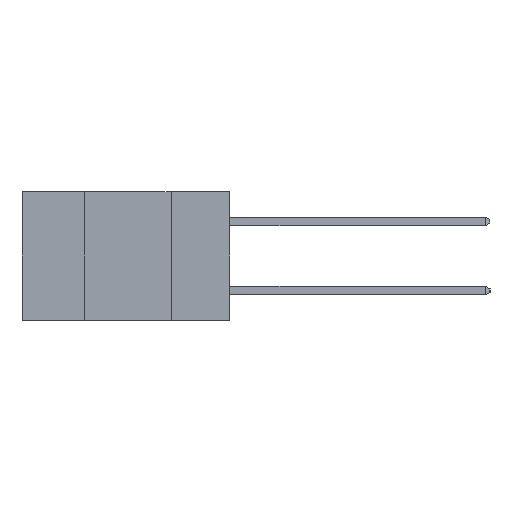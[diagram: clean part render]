
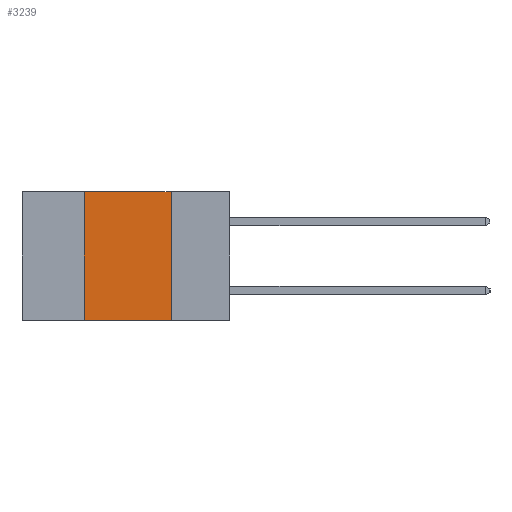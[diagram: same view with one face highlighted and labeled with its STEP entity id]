
A CAD part, left-side view. The second image highlights one B-rep face of the part: STEP entity #3239.
In plain terms, the highlighted planar face has unit normal (-1, 0, 0).
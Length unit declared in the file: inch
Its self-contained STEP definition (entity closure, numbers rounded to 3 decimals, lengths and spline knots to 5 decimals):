
#440 = CARTESIAN_POINT ( 'NONE',  ( 0., 0.42, 0. ) ) ;
#556 = DIRECTION ( 'NONE',  ( 0., 0., 1. ) ) ;
#695 = EDGE_CURVE ( 'NONE', #1927, #7465, #1790, .T. ) ;
#771 = CARTESIAN_POINT ( 'NONE',  ( 0., 0.6, 0. ) ) ;
#850 = VERTEX_POINT ( 'NONE', #440 ) ;
#867 = DIRECTION ( 'NONE',  ( 0., -1., 0. ) ) ;
#1201 = EDGE_CURVE ( 'NONE', #8015, #7465, #5450, .T. ) ;
#1234 = CARTESIAN_POINT ( 'NONE',  ( 0., 0.6, -0.37 ) ) ;
#1240 = VECTOR ( 'NONE', #5137, 39.37008 ) ;
#1754 = LINE ( 'NONE', #10065, #10450 ) ;
#1790 = LINE ( 'NONE', #3501, #1240 ) ;
#1927 = VERTEX_POINT ( 'NONE', #2365 ) ;
#2286 = EDGE_CURVE ( 'NONE', #8015, #850, #1754, .T. ) ;
#2365 = CARTESIAN_POINT ( 'NONE',  ( 0., 0.17, 0. ) ) ;
#3239 = ADVANCED_FACE ( 'NONE', ( #10012 ), #7728, .F. ) ;
#3389 = VECTOR ( 'NONE', #867, 39.37008 ) ;
#3501 = CARTESIAN_POINT ( 'NONE',  ( 0., 0.17, -0.37 ) ) ;
#3591 = CARTESIAN_POINT ( 'NONE',  ( 0., 0.17, -0.37 ) ) ;
#4208 = LINE ( 'NONE', #8616, #3389 ) ;
#4682 = EDGE_LOOP ( 'NONE', ( #9086, #4847, #5423, #8098 ) ) ;
#4711 = DIRECTION ( 'NONE',  ( 0., -1., 0. ) ) ;
#4847 = ORIENTED_EDGE ( 'NONE', *, *, #8706, .F. ) ;
#5137 = DIRECTION ( 'NONE',  ( 0., 0., -1. ) ) ;
#5423 = ORIENTED_EDGE ( 'NONE', *, *, #2286, .F. ) ;
#5450 = LINE ( 'NONE', #1234, #9801 ) ;
#7465 = VERTEX_POINT ( 'NONE', #3591 ) ;
#7728 = PLANE ( 'NONE',  #8981 ) ;
#8015 = VERTEX_POINT ( 'NONE', #9256 ) ;
#8098 = ORIENTED_EDGE ( 'NONE', *, *, #1201, .T. ) ;
#8616 = CARTESIAN_POINT ( 'NONE',  ( 0., 0.6, 0. ) ) ;
#8706 = EDGE_CURVE ( 'NONE', #850, #1927, #4208, .T. ) ;
#8981 = AXIS2_PLACEMENT_3D ( 'NONE', #771, #10322, #10359 ) ;
#9086 = ORIENTED_EDGE ( 'NONE', *, *, #695, .F. ) ;
#9256 = CARTESIAN_POINT ( 'NONE',  ( 0., 0.42, -0.37 ) ) ;
#9801 = VECTOR ( 'NONE', #4711, 39.37008 ) ;
#10012 = FACE_OUTER_BOUND ( 'NONE', #4682, .T. ) ;
#10065 = CARTESIAN_POINT ( 'NONE',  ( 0., 0.42, -0.37 ) ) ;
#10322 = DIRECTION ( 'NONE',  ( 1., 0., 0. ) ) ;
#10359 = DIRECTION ( 'NONE',  ( 0., 0., -1. ) ) ;
#10450 = VECTOR ( 'NONE', #556, 39.37008 ) ;
